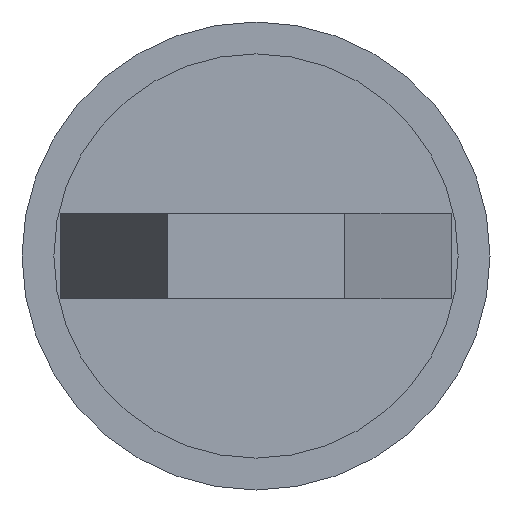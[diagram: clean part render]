
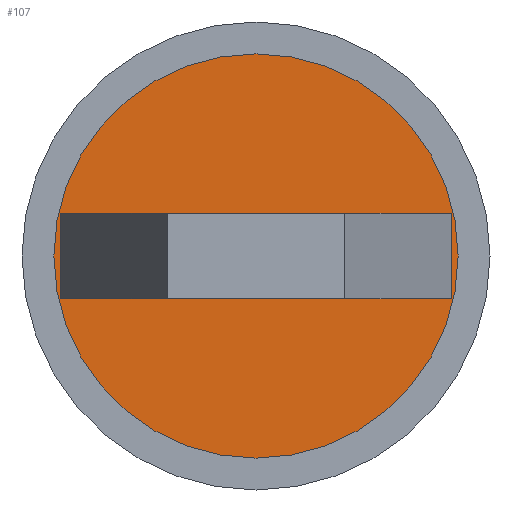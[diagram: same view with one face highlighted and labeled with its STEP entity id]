
A CAD part, left-side view. The second image highlights one B-rep face of the part: STEP entity #107.
In plain terms, the highlighted planar face has unit normal (-1, 0, 0).
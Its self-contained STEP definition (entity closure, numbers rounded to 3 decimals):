
#5 = CARTESIAN_POINT ( 'NONE',  ( -211.682, 37.343, 1. ) ) ;
#10 = CIRCLE ( 'NONE', #93, 9.5 ) ;
#21 = CARTESIAN_POINT ( 'NONE',  ( -211.682, 46.521, 1. ) ) ;
#38 = CARTESIAN_POINT ( 'NONE',  ( -211.682, 56.021, 1. ) ) ;
#41 = VECTOR ( 'NONE', #349, 1000. ) ;
#47 = VERTEX_POINT ( 'NONE', #214 ) ;
#48 = LINE ( 'NONE', #400, #104 ) ;
#63 = CARTESIAN_POINT ( 'NONE',  ( -211.682, 46.521, 1. ) ) ;
#90 = EDGE_CURVE ( 'NONE', #274, #215, #10, .T. ) ;
#93 = AXIS2_PLACEMENT_3D ( 'NONE', #63, #170, #218 ) ;
#104 = VECTOR ( 'NONE', #403, 1000. ) ;
#107 = ADVANCED_FACE ( 'NONE', ( #364, #553 ), #415, .T. ) ;
#118 = DIRECTION ( 'NONE',  ( 0., -1., 0. ) ) ;
#125 = ORIENTED_EDGE ( 'NONE', *, *, #90, .F. ) ;
#127 = DIRECTION ( 'NONE',  ( 0., -1., 0. ) ) ;
#170 = DIRECTION ( 'NONE',  ( 1., 0., 0. ) ) ;
#214 = CARTESIAN_POINT ( 'NONE',  ( -211.682, 37.343, -1. ) ) ;
#215 = VERTEX_POINT ( 'NONE', #38 ) ;
#218 = DIRECTION ( 'NONE',  ( 0., -1., 0. ) ) ;
#231 = AXIS2_PLACEMENT_3D ( 'NONE', #464, #359, #614 ) ;
#251 = LINE ( 'NONE', #5, #41 ) ;
#265 = AXIS2_PLACEMENT_3D ( 'NONE', #21, #607, #118 ) ;
#268 = CARTESIAN_POINT ( 'NONE',  ( -211.682, 46.521, 3. ) ) ;
#274 = VERTEX_POINT ( 'NONE', #452 ) ;
#280 = VECTOR ( 'NONE', #492, 1000. ) ;
#283 = ORIENTED_EDGE ( 'NONE', *, *, #378, .T. ) ;
#293 = ORIENTED_EDGE ( 'NONE', *, *, #567, .T. ) ;
#298 = EDGE_CURVE ( 'NONE', #348, #47, #251, .T. ) ;
#324 = ORIENTED_EDGE ( 'NONE', *, *, #298, .T. ) ;
#340 = VERTEX_POINT ( 'NONE', #405 ) ;
#341 = EDGE_CURVE ( 'NONE', #372, #340, #48, .T. ) ;
#348 = VERTEX_POINT ( 'NONE', #541 ) ;
#349 = DIRECTION ( 'NONE',  ( 0., 0., -1. ) ) ;
#351 = ORIENTED_EDGE ( 'NONE', *, *, #431, .F. ) ;
#359 = DIRECTION ( 'NONE',  ( 1., 0., 0. ) ) ;
#361 = VECTOR ( 'NONE', #127, 1000. ) ;
#364 = FACE_BOUND ( 'NONE', #572, .T. ) ;
#372 = VERTEX_POINT ( 'NONE', #495 ) ;
#378 = EDGE_CURVE ( 'NONE', #47, #372, #595, .T. ) ;
#389 = EDGE_LOOP ( 'NONE', ( #125, #351 ) ) ;
#399 = ORIENTED_EDGE ( 'NONE', *, *, #341, .T. ) ;
#400 = CARTESIAN_POINT ( 'NONE',  ( -211.682, 55.699, 1. ) ) ;
#403 = DIRECTION ( 'NONE',  ( 0., 0., 1. ) ) ;
#405 = CARTESIAN_POINT ( 'NONE',  ( -211.682, 55.699, 3. ) ) ;
#415 = PLANE ( 'NONE',  #265 ) ;
#431 = EDGE_CURVE ( 'NONE', #215, #274, #573, .T. ) ;
#452 = CARTESIAN_POINT ( 'NONE',  ( -211.682, 37.021, 1. ) ) ;
#464 = CARTESIAN_POINT ( 'NONE',  ( -211.682, 46.521, 1. ) ) ;
#492 = DIRECTION ( 'NONE',  ( 0., 1., 0. ) ) ;
#495 = CARTESIAN_POINT ( 'NONE',  ( -211.682, 55.699, -1. ) ) ;
#511 = LINE ( 'NONE', #268, #361 ) ;
#537 = CARTESIAN_POINT ( 'NONE',  ( -211.682, 46.521, -1. ) ) ;
#541 = CARTESIAN_POINT ( 'NONE',  ( -211.682, 37.343, 3. ) ) ;
#553 = FACE_OUTER_BOUND ( 'NONE', #389, .T. ) ;
#567 = EDGE_CURVE ( 'NONE', #340, #348, #511, .T. ) ;
#572 = EDGE_LOOP ( 'NONE', ( #399, #293, #324, #283 ) ) ;
#573 = CIRCLE ( 'NONE', #231, 9.5 ) ;
#595 = LINE ( 'NONE', #537, #280 ) ;
#607 = DIRECTION ( 'NONE',  ( -1., 0., 0. ) ) ;
#614 = DIRECTION ( 'NONE',  ( 0., -1., 0. ) ) ;
